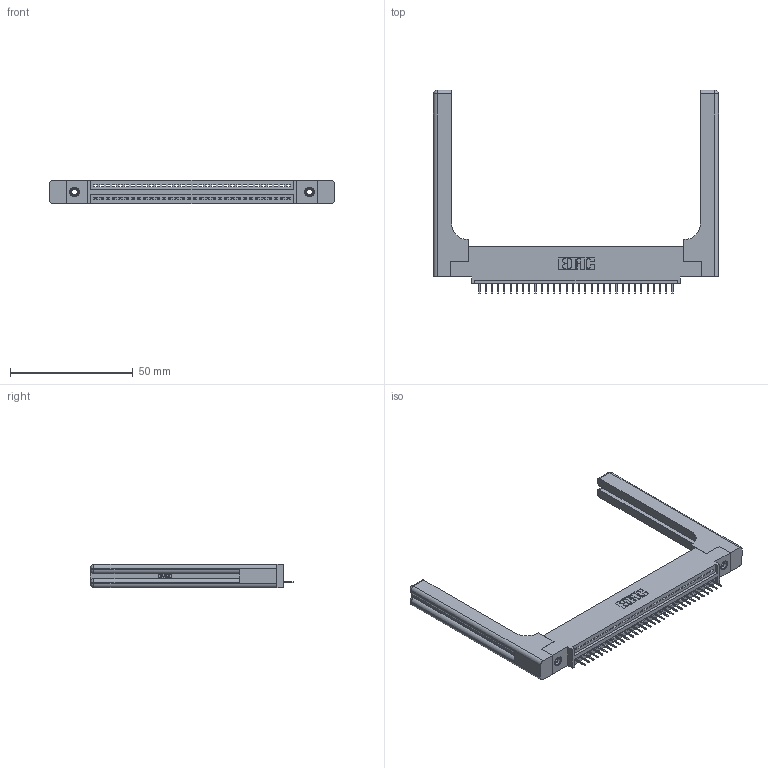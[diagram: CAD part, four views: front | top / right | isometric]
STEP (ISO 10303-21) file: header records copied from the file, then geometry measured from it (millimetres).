
FILE_DESCRIPTION (( 'STEP AP203' ), '1' );
FILE_NAME ('345-032-524-458.STEP', '2019-10-07T14:11:41', ( '' ), ( '' ), 'SwSTEP 2.0', 'SolidWorks 2016', '' );
FILE_SCHEMA (( 'CONFIG_CONTROL_DESIGN' ));
Length unit declared in the file: inch
Products named in the file (5): 345-250-001_345-250-001-102; 345-220-058_345-220-058; 345-032-524-458; 345-292-001_345-293-124; 345 Part_0.110 Offset - 0.156 Dia-TH
Assembly tree (37 placements, depth 2):
  345-032-524-458
    345 Part_0.110 Offset - 0.156 Dia-TH
    345-292-001_345-293-124  x32
    345-250-001_345-250-001-102  x2
    345-220-058_345-220-058  x2
Bounding box: 116.31 x 83.11 x 9.4 mm (x, y, z)
Volume: 19270.2 mm3; surface area: 19153.4 mm2
Topology: 37 solids, 37 shells, 2370 faces, 6779 edges, 4370 vertices
Faces by surface type: plane 1704, cylinder 606, bspline 36, cone 12, sphere 8, torus 4
Entity records: 30818 total; most frequent: CARTESIAN_POINT 6309, ORIENTED_EDGE 5072, DIRECTION 4472, EDGE_CURVE 2536, LINE 2188, VECTOR 2188, VERTEX_POINT 1678, AXIS2_PLACEMENT_3D 1142
